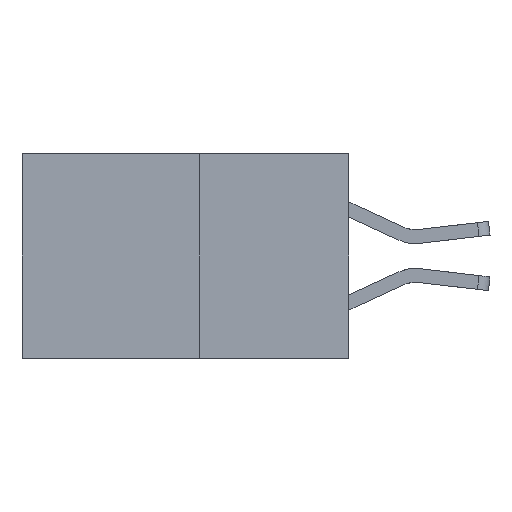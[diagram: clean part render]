
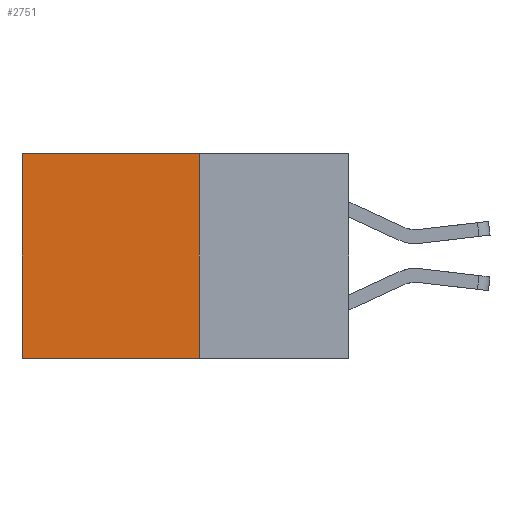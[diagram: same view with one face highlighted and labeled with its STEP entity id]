
A CAD part, left-side view. The second image highlights one B-rep face of the part: STEP entity #2751.
In plain terms, the highlighted planar face has unit normal (-1, 0, 0).
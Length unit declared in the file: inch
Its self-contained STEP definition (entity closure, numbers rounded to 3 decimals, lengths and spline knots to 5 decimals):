
#6 = ORIENTED_EDGE ( 'NONE', *, *, #6826, .F. ) ;
#28 = ORIENTED_EDGE ( 'NONE', *, *, #6234, .F. ) ;
#38 = ORIENTED_EDGE ( 'NONE', *, *, #4845, .T. ) ;
#71 = CARTESIAN_POINT ( 'NONE',  ( 0.277, 0.59, -0.37 ) ) ;
#91 = CARTESIAN_POINT ( 'NONE',  ( 0.277, 0.27, -0.37 ) ) ;
#651 = VECTOR ( 'NONE', #2550, 39.37008 ) ;
#743 = VERTEX_POINT ( 'NONE', #7750 ) ;
#1256 = FACE_OUTER_BOUND ( 'NONE', #1425, .T. ) ;
#1425 = EDGE_LOOP ( 'NONE', ( #38, #28, #6, #4703 ) ) ;
#1593 = VERTEX_POINT ( 'NONE', #3290 ) ;
#2213 = PLANE ( 'NONE',  #4396 ) ;
#2550 = DIRECTION ( 'NONE',  ( 0., 1., 0. ) ) ;
#2595 = VECTOR ( 'NONE', #3260, 39.37008 ) ;
#2655 = CARTESIAN_POINT ( 'NONE',  ( 0.277, 0.27, 0. ) ) ;
#2690 = LINE ( 'NONE', #91, #651 ) ;
#2751 = ADVANCED_FACE ( 'NONE', ( #1256 ), #2213, .F. ) ;
#2920 = EDGE_CURVE ( 'NONE', #743, #1593, #6762, .T. ) ;
#3260 = DIRECTION ( 'NONE',  ( 0., 0., -1. ) ) ;
#3290 = CARTESIAN_POINT ( 'NONE',  ( 0.277, 0.59, 0. ) ) ;
#3474 = DIRECTION ( 'NONE',  ( 1., 0., 0. ) ) ;
#4396 = AXIS2_PLACEMENT_3D ( 'NONE', #7749, #3474, #7398 ) ;
#4703 = ORIENTED_EDGE ( 'NONE', *, *, #2920, .T. ) ;
#4726 = VECTOR ( 'NONE', #8075, 39.37008 ) ;
#4845 = EDGE_CURVE ( 'NONE', #1593, #7301, #6669, .T. ) ;
#5545 = CARTESIAN_POINT ( 'NONE',  ( 0.277, 0.27, -0.37 ) ) ;
#5692 = VECTOR ( 'NONE', #8694, 39.37008 ) ;
#6015 = CARTESIAN_POINT ( 'NONE',  ( 0.277, 0.59, -0.37 ) ) ;
#6234 = EDGE_CURVE ( 'NONE', #8054, #7301, #2690, .T. ) ;
#6669 = LINE ( 'NONE', #71, #2595 ) ;
#6762 = LINE ( 'NONE', #2655, #4726 ) ;
#6826 = EDGE_CURVE ( 'NONE', #743, #8054, #7448, .T. ) ;
#6845 = CARTESIAN_POINT ( 'NONE',  ( 0.277, 0.27, -0.37 ) ) ;
#7301 = VERTEX_POINT ( 'NONE', #6015 ) ;
#7398 = DIRECTION ( 'NONE',  ( 0., 0., -1. ) ) ;
#7448 = LINE ( 'NONE', #6845, #5692 ) ;
#7749 = CARTESIAN_POINT ( 'NONE',  ( 0.277, 0.27, -0.37 ) ) ;
#7750 = CARTESIAN_POINT ( 'NONE',  ( 0.277, 0.27, 0. ) ) ;
#8054 = VERTEX_POINT ( 'NONE', #5545 ) ;
#8075 = DIRECTION ( 'NONE',  ( 0., 1., 0. ) ) ;
#8694 = DIRECTION ( 'NONE',  ( 0., 0., -1. ) ) ;
